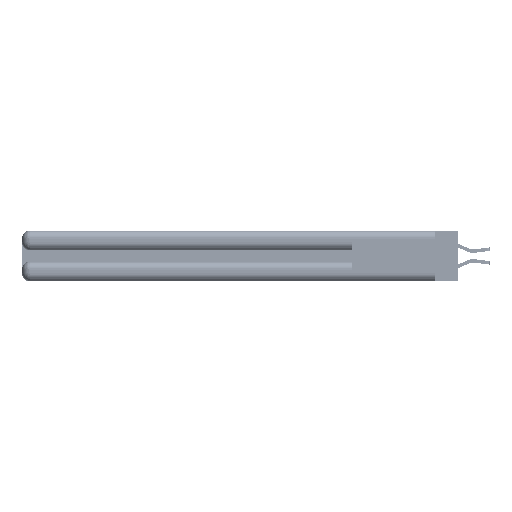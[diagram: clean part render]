
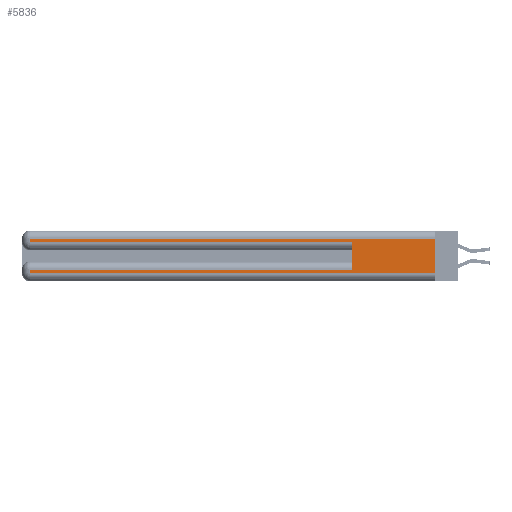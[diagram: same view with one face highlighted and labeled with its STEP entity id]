
A CAD part, left-side view. The second image highlights one B-rep face of the part: STEP entity #5836.
In plain terms, the highlighted planar face has unit normal (-1, 0, 0).
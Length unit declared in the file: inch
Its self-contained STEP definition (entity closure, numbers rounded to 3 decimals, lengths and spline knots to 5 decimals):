
#892 = ORIENTED_EDGE ( 'NONE', *, *, #27709, .T. ) ;
#1292 = CARTESIAN_POINT ( 'NONE',  ( 0., 2.94, 0.085 ) ) ;
#3427 = VECTOR ( 'NONE', #54709, 39.37008 ) ;
#3476 = DIRECTION ( 'NONE',  ( 1., 0., 0. ) ) ;
#4461 = DIRECTION ( 'NONE',  ( 0., 0., -1. ) ) ;
#5309 = VECTOR ( 'NONE', #22920, 39.37008 ) ;
#5836 = ADVANCED_FACE ( 'NONE', ( #40555 ), #30043, .F. ) ;
#6239 = LINE ( 'NONE', #50239, #3427 ) ;
#7034 = CARTESIAN_POINT ( 'NONE',  ( 0., 0., 0.37 ) ) ;
#7678 = VERTEX_POINT ( 'NONE', #52705 ) ;
#8179 = CARTESIAN_POINT ( 'NONE',  ( 0., 0.6, 0.285 ) ) ;
#8645 = CARTESIAN_POINT ( 'NONE',  ( 0., 2.94, 0.37 ) ) ;
#8650 = VERTEX_POINT ( 'NONE', #37068 ) ;
#8955 = CARTESIAN_POINT ( 'NONE',  ( 0., 2.94, 0.37 ) ) ;
#9035 = EDGE_CURVE ( 'NONE', #41155, #57288, #6239, .T. ) ;
#10331 = AXIS2_PLACEMENT_3D ( 'NONE', #56644, #3476, #34501 ) ;
#11491 = CARTESIAN_POINT ( 'NONE',  ( 0., 0.6, 0.085 ) ) ;
#13719 = CARTESIAN_POINT ( 'NONE',  ( 0., 2.94, 0.31 ) ) ;
#14169 = ORIENTED_EDGE ( 'NONE', *, *, #39215, .F. ) ;
#14231 = VECTOR ( 'NONE', #4461, 39.37008 ) ;
#14245 = VERTEX_POINT ( 'NONE', #48261 ) ;
#14494 = VERTEX_POINT ( 'NONE', #1292 ) ;
#14980 = DIRECTION ( 'NONE',  ( 0., 1., 0. ) ) ;
#15621 = LINE ( 'NONE', #8955, #14231 ) ;
#17093 = LINE ( 'NONE', #18450, #5309 ) ;
#17540 = DIRECTION ( 'NONE',  ( 0., 0., -1. ) ) ;
#18450 = CARTESIAN_POINT ( 'NONE',  ( 0., 0., 0.285 ) ) ;
#20393 = DIRECTION ( 'NONE',  ( 0., 0., -1. ) ) ;
#21225 = LINE ( 'NONE', #8645, #55222 ) ;
#21908 = CARTESIAN_POINT ( 'NONE',  ( 0., 0., 0.06 ) ) ;
#22621 = ORIENTED_EDGE ( 'NONE', *, *, #25796, .T. ) ;
#22920 = DIRECTION ( 'NONE',  ( 0., -1., 0. ) ) ;
#24264 = VECTOR ( 'NONE', #30788, 39.37008 ) ;
#25796 = EDGE_CURVE ( 'NONE', #41155, #14494, #52229, .T. ) ;
#27157 = ORIENTED_EDGE ( 'NONE', *, *, #47143, .T. ) ;
#27709 = EDGE_CURVE ( 'NONE', #42250, #7678, #15621, .T. ) ;
#27951 = ORIENTED_EDGE ( 'NONE', *, *, #33835, .T. ) ;
#28364 = CARTESIAN_POINT ( 'NONE',  ( 0., 0., 0.31 ) ) ;
#28377 = CARTESIAN_POINT ( 'NONE',  ( 0., 0., 0.31 ) ) ;
#28720 = VECTOR ( 'NONE', #14980, 39.37008 ) ;
#29109 = VERTEX_POINT ( 'NONE', #28377 ) ;
#30043 = PLANE ( 'NONE',  #10331 ) ;
#30177 = EDGE_LOOP ( 'NONE', ( #14169, #34764, #892, #27157, #31649, #22621, #49317, #27951 ) ) ;
#30788 = DIRECTION ( 'NONE',  ( 0., -1., 0. ) ) ;
#31649 = ORIENTED_EDGE ( 'NONE', *, *, #9035, .F. ) ;
#33810 = VECTOR ( 'NONE', #20393, 39.37008 ) ;
#33835 = EDGE_CURVE ( 'NONE', #14245, #8650, #36074, .T. ) ;
#34501 = DIRECTION ( 'NONE',  ( 0., 0., -1. ) ) ;
#34764 = ORIENTED_EDGE ( 'NONE', *, *, #53172, .T. ) ;
#35954 = DIRECTION ( 'NONE',  ( 0., 1., 0. ) ) ;
#36074 = LINE ( 'NONE', #21908, #24264 ) ;
#37068 = CARTESIAN_POINT ( 'NONE',  ( 0., 0., 0.06 ) ) ;
#39215 = EDGE_CURVE ( 'NONE', #29109, #8650, #57466, .T. ) ;
#40506 = LINE ( 'NONE', #28364, #28720 ) ;
#40555 = FACE_OUTER_BOUND ( 'NONE', #30177, .T. ) ;
#41155 = VERTEX_POINT ( 'NONE', #11491 ) ;
#42250 = VERTEX_POINT ( 'NONE', #13719 ) ;
#47143 = EDGE_CURVE ( 'NONE', #7678, #57288, #17093, .T. ) ;
#48230 = EDGE_CURVE ( 'NONE', #14494, #14245, #21225, .T. ) ;
#48261 = CARTESIAN_POINT ( 'NONE',  ( 0., 2.94, 0.06 ) ) ;
#49317 = ORIENTED_EDGE ( 'NONE', *, *, #48230, .T. ) ;
#49321 = CARTESIAN_POINT ( 'NONE',  ( 0., 0., 0.085 ) ) ;
#49444 = VECTOR ( 'NONE', #35954, 39.37008 ) ;
#50239 = CARTESIAN_POINT ( 'NONE',  ( 0., 0.6, 0.145 ) ) ;
#52229 = LINE ( 'NONE', #49321, #49444 ) ;
#52705 = CARTESIAN_POINT ( 'NONE',  ( 0., 2.94, 0.285 ) ) ;
#53172 = EDGE_CURVE ( 'NONE', #29109, #42250, #40506, .T. ) ;
#54709 = DIRECTION ( 'NONE',  ( 0., 0., 1. ) ) ;
#55222 = VECTOR ( 'NONE', #17540, 39.37008 ) ;
#56644 = CARTESIAN_POINT ( 'NONE',  ( 0., 0., 0.37 ) ) ;
#57288 = VERTEX_POINT ( 'NONE', #8179 ) ;
#57466 = LINE ( 'NONE', #7034, #33810 ) ;
